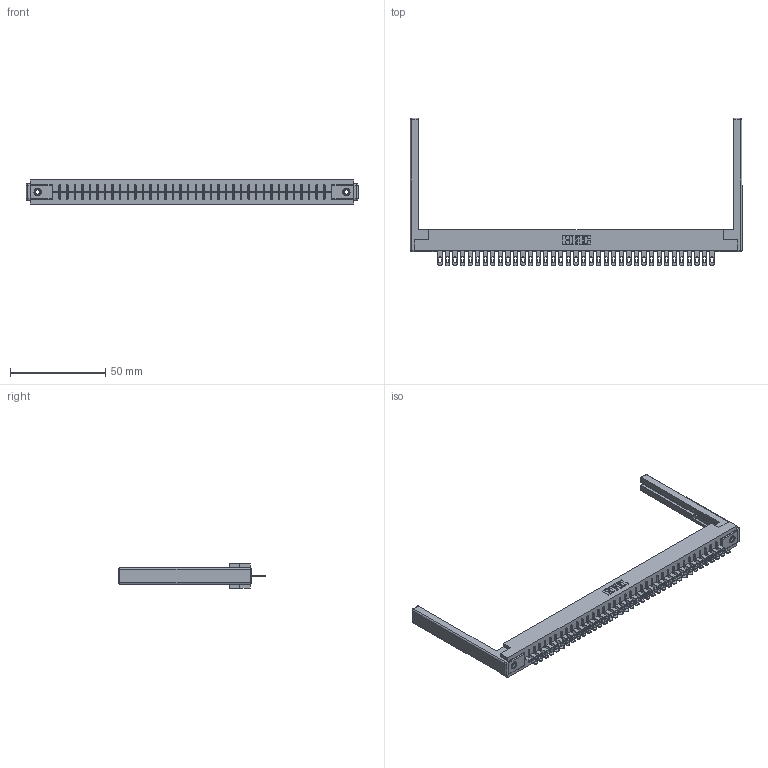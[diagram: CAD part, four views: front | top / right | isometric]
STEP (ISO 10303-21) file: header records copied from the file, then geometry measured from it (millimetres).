
FILE_DESCRIPTION (( 'STEP AP203' ), '1' );
FILE_NAME ('306-037-400-168.STEP', '2020-09-22T04:54:11', ( '' ), ( '' ), 'SwSTEP 2.0', 'SolidWorks 2020', '' );
FILE_SCHEMA (( 'CONFIG_CONTROL_DESIGN' ));
Length unit declared in the file: inch
Products named in the file (5): 307-220-068; 345-250-001_345-250-001-102; 306-037-400-168; 306-290-001_100; 306 Part_.156 Dia
Assembly tree (42 placements, depth 2):
  306-037-400-168
    306 Part_.156 Dia
    306-290-001_100  x37
    345-250-001_345-250-001-102  x2
    307-220-068  x2
Bounding box: 174.04 x 77.17 x 12.7 mm (x, y, z)
Volume: 23681.1 mm3; surface area: 24489.6 mm2
Topology: 42 solids, 42 shells, 3082 faces, 8661 edges, 5554 vertices
Faces by surface type: plane 2006, cylinder 904, sphere 156, cone 12, torus 4
Entity records: 38075 total; most frequent: CARTESIAN_POINT 6359, ORIENTED_EDGE 6296, DIRECTION 6284, EDGE_CURVE 3148, VECTOR 2454, LINE 2454, VERTEX_POINT 1990, AXIS2_PLACEMENT_3D 1915
